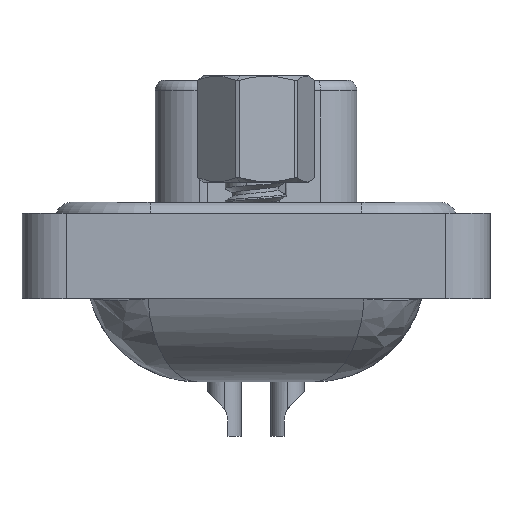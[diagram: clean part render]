
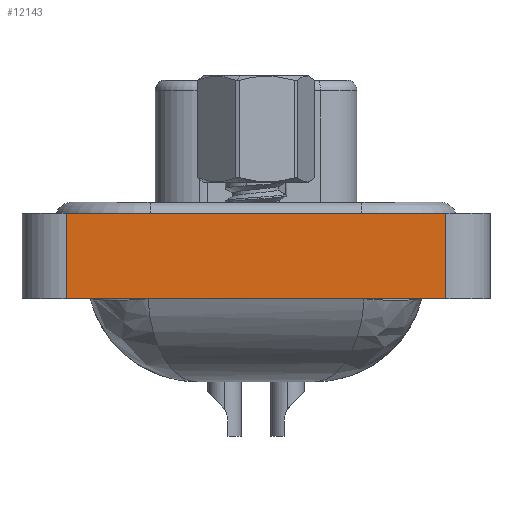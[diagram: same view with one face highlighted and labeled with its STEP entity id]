
A CAD part, left-side view. The second image highlights one B-rep face of the part: STEP entity #12143.
In plain terms, the highlighted planar face has unit normal (-1, 0, 0).
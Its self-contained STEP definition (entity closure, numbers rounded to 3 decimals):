
#1334 = VECTOR ( 'NONE', #7323, 1000. ) ;
#1852 = EDGE_CURVE ( 'NONE', #4284, #4704, #3112, .T. ) ;
#1860 = DIRECTION ( 'NONE',  ( -1., 0., 0. ) ) ;
#2279 = DIRECTION ( 'NONE',  ( 0., 0., 1. ) ) ;
#3112 = LINE ( 'NONE', #14289, #17527 ) ;
#4089 = CARTESIAN_POINT ( 'NONE',  ( -7.25, -8.55, 0.5 ) ) ;
#4284 = VERTEX_POINT ( 'NONE', #19846 ) ;
#4454 = LINE ( 'NONE', #16941, #1334 ) ;
#4611 = EDGE_CURVE ( 'NONE', #4704, #10569, #13056, .T. ) ;
#4704 = VERTEX_POINT ( 'NONE', #12221 ) ;
#6471 = FACE_OUTER_BOUND ( 'NONE', #19657, .T. ) ;
#6506 = ORIENTED_EDGE ( 'NONE', *, *, #13872, .F. ) ;
#6788 = CARTESIAN_POINT ( 'NONE',  ( -7.25, 8.55, -3.35 ) ) ;
#6897 = DIRECTION ( 'NONE',  ( 0., 0., 1. ) ) ;
#7323 = DIRECTION ( 'NONE',  ( 0., -1., 0. ) ) ;
#8122 = PLANE ( 'NONE',  #14054 ) ;
#8750 = ORIENTED_EDGE ( 'NONE', *, *, #14236, .F. ) ;
#10569 = VERTEX_POINT ( 'NONE', #4089 ) ;
#11206 = DIRECTION ( 'NONE',  ( 0., -1., 0. ) ) ;
#12143 = ADVANCED_FACE ( 'NONE', ( #6471 ), #8122, .T. ) ;
#12221 = CARTESIAN_POINT ( 'NONE',  ( -7.25, -8.55, -3.35 ) ) ;
#13056 = LINE ( 'NONE', #14698, #17762 ) ;
#13248 = LINE ( 'NONE', #6788, #16403 ) ;
#13863 = ORIENTED_EDGE ( 'NONE', *, *, #1852, .T. ) ;
#13872 = EDGE_CURVE ( 'NONE', #19472, #10569, #4454, .T. ) ;
#13918 = CARTESIAN_POINT ( 'NONE',  ( -7.25, 8.55, 0.5 ) ) ;
#14054 = AXIS2_PLACEMENT_3D ( 'NONE', #16104, #1860, #19302 ) ;
#14236 = EDGE_CURVE ( 'NONE', #4284, #19472, #13248, .T. ) ;
#14289 = CARTESIAN_POINT ( 'NONE',  ( -7.25, -8.55, -3.35 ) ) ;
#14698 = CARTESIAN_POINT ( 'NONE',  ( -7.25, -8.55, -3.35 ) ) ;
#16104 = CARTESIAN_POINT ( 'NONE',  ( -7.25, -8.55, -3.35 ) ) ;
#16403 = VECTOR ( 'NONE', #2279, 1000. ) ;
#16941 = CARTESIAN_POINT ( 'NONE',  ( -7.25, -8.55, 0.5 ) ) ;
#17527 = VECTOR ( 'NONE', #11206, 1000. ) ;
#17762 = VECTOR ( 'NONE', #6897, 1000. ) ;
#18926 = ORIENTED_EDGE ( 'NONE', *, *, #4611, .T. ) ;
#19302 = DIRECTION ( 'NONE',  ( 0., 0., 1. ) ) ;
#19472 = VERTEX_POINT ( 'NONE', #13918 ) ;
#19657 = EDGE_LOOP ( 'NONE', ( #18926, #6506, #8750, #13863 ) ) ;
#19846 = CARTESIAN_POINT ( 'NONE',  ( -7.25, 8.55, -3.35 ) ) ;
